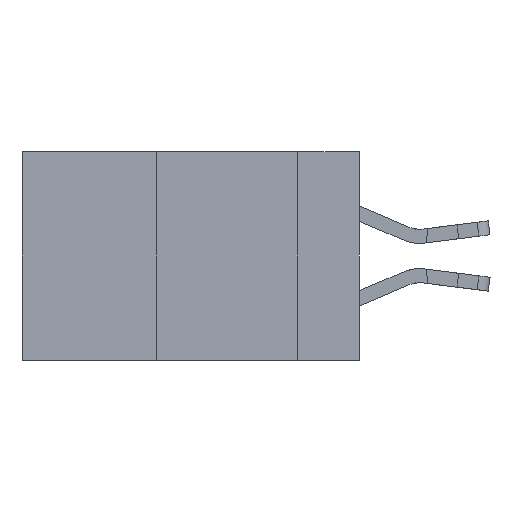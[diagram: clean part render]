
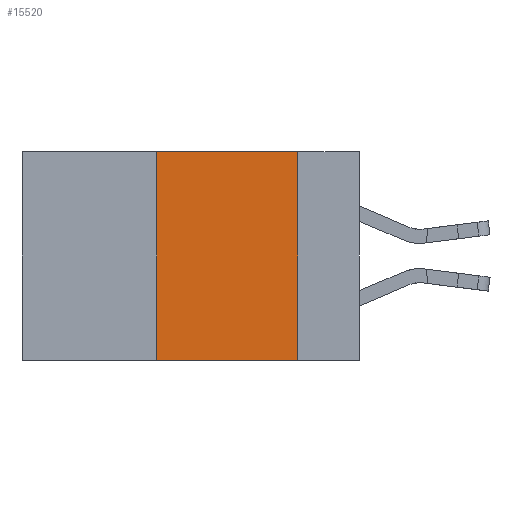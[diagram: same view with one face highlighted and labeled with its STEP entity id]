
A CAD part, left-side view. The second image highlights one B-rep face of the part: STEP entity #15520.
In plain terms, the highlighted planar face has unit normal (-1, 0, 0).
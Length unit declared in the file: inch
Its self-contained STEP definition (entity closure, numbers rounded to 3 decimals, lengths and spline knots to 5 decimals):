
#286 = ORIENTED_EDGE ( 'NONE', *, *, #22885, .F. ) ;
#1424 = AXIS2_PLACEMENT_3D ( 'NONE', #1562, #3383, #15802 ) ;
#1562 = CARTESIAN_POINT ( 'NONE',  ( 0., 0.6, 0. ) ) ;
#2916 = DIRECTION ( 'NONE',  ( 0., -1., 0. ) ) ;
#2954 = DIRECTION ( 'NONE',  ( 0., 0., 1. ) ) ;
#3006 = VERTEX_POINT ( 'NONE', #5092 ) ;
#3164 = ORIENTED_EDGE ( 'NONE', *, *, #18314, .T. ) ;
#3296 = EDGE_CURVE ( 'NONE', #6661, #10525, #19504, .T. ) ;
#3383 = DIRECTION ( 'NONE',  ( 1., 0., 0. ) ) ;
#4092 = CARTESIAN_POINT ( 'NONE',  ( 0., 0.36, -0.37 ) ) ;
#5092 = CARTESIAN_POINT ( 'NONE',  ( 0., 0.36, 0. ) ) ;
#5297 = CARTESIAN_POINT ( 'NONE',  ( 0., 0.11, -0.37 ) ) ;
#6365 = VECTOR ( 'NONE', #18557, 39.37008 ) ;
#6661 = VERTEX_POINT ( 'NONE', #16947 ) ;
#7298 = ORIENTED_EDGE ( 'NONE', *, *, #3296, .F. ) ;
#9427 = FACE_OUTER_BOUND ( 'NONE', #18585, .T. ) ;
#10077 = VERTEX_POINT ( 'NONE', #4092 ) ;
#10525 = VERTEX_POINT ( 'NONE', #5297 ) ;
#11001 = VECTOR ( 'NONE', #2916, 39.37008 ) ;
#11152 = LINE ( 'NONE', #11596, #6365 ) ;
#11558 = LINE ( 'NONE', #18796, #11001 ) ;
#11596 = CARTESIAN_POINT ( 'NONE',  ( 0., 0.6, 0. ) ) ;
#13443 = CARTESIAN_POINT ( 'NONE',  ( 0., 0.11, 0. ) ) ;
#13622 = CARTESIAN_POINT ( 'NONE',  ( 0., 0.36, 0. ) ) ;
#15187 = VECTOR ( 'NONE', #18581, 39.37008 ) ;
#15520 = ADVANCED_FACE ( 'NONE', ( #9427 ), #20880, .F. ) ;
#15802 = DIRECTION ( 'NONE',  ( 0., 0., -1. ) ) ;
#16947 = CARTESIAN_POINT ( 'NONE',  ( 0., 0.11, 0. ) ) ;
#18314 = EDGE_CURVE ( 'NONE', #10077, #10525, #11558, .T. ) ;
#18557 = DIRECTION ( 'NONE',  ( 0., -1., 0. ) ) ;
#18581 = DIRECTION ( 'NONE',  ( 0., 0., -1. ) ) ;
#18585 = EDGE_LOOP ( 'NONE', ( #7298, #18862, #286, #3164 ) ) ;
#18796 = CARTESIAN_POINT ( 'NONE',  ( 0., 0.6, -0.37 ) ) ;
#18862 = ORIENTED_EDGE ( 'NONE', *, *, #20675, .F. ) ;
#19504 = LINE ( 'NONE', #13443, #15187 ) ;
#20675 = EDGE_CURVE ( 'NONE', #3006, #6661, #11152, .T. ) ;
#20880 = PLANE ( 'NONE',  #1424 ) ;
#21889 = LINE ( 'NONE', #13622, #22410 ) ;
#22410 = VECTOR ( 'NONE', #2954, 39.37008 ) ;
#22885 = EDGE_CURVE ( 'NONE', #10077, #3006, #21889, .T. ) ;
